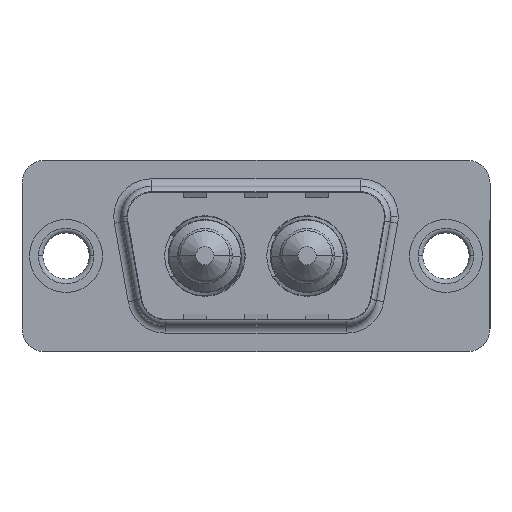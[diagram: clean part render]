
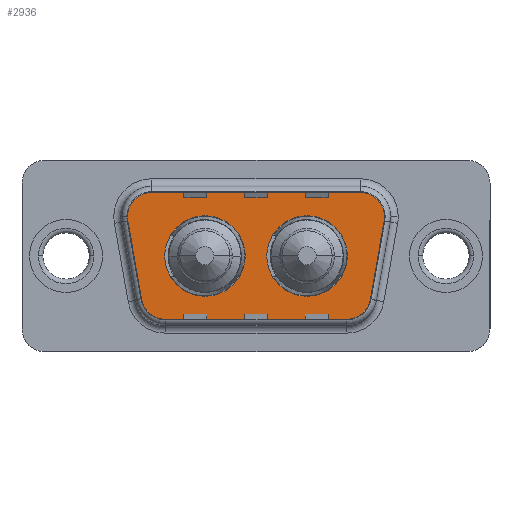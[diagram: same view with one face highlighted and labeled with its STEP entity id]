
A CAD part, top view. The second image highlights one B-rep face of the part: STEP entity #2936.
In plain terms, the highlighted planar face has unit normal (0, 0, 1).
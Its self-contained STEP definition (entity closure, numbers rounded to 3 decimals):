
#11 = CARTESIAN_POINT ( 'NONE',  ( 6.49, 0., 0. ) ) ;
#120 = CIRCLE ( 'NONE', #6072, 2. ) ;
#164 = VERTEX_POINT ( 'NONE', #4654 ) ;
#494 = DIRECTION ( 'NONE',  ( 0., 0., 1. ) ) ;
#540 = CARTESIAN_POINT ( 'NONE',  ( 21.564, 2.9, 0. ) ) ;
#599 = ORIENTED_EDGE ( 'NONE', *, *, #8044, .T. ) ;
#645 = DIRECTION ( 'NONE',  ( 0.174, -0.985, 0. ) ) ;
#717 = DIRECTION ( 'NONE',  ( 1., 0., 0. ) ) ;
#745 = CARTESIAN_POINT ( 'NONE',  ( 18.541, -2.9, 0. ) ) ;
#781 = DIRECTION ( 'NONE',  ( 0., 0., 1. ) ) ;
#797 = DIRECTION ( 'NONE',  ( 1., 0., 0. ) ) ;
#807 = CARTESIAN_POINT ( 'NONE',  ( 5.436, 2.9, 0. ) ) ;
#845 = ORIENTED_EDGE ( 'NONE', *, *, #3369, .T. ) ;
#969 = AXIS2_PLACEMENT_3D ( 'NONE', #7450, #4734, #2533 ) ;
#1001 = VERTEX_POINT ( 'NONE', #7862 ) ;
#1220 = DIRECTION ( 'NONE',  ( 0., 0., 1. ) ) ;
#1245 = ORIENTED_EDGE ( 'NONE', *, *, #6225, .T. ) ;
#1254 = EDGE_LOOP ( 'NONE', ( #5121, #5214 ) ) ;
#1311 = AXIS2_PLACEMENT_3D ( 'NONE', #7008, #5118, #5617 ) ;
#1344 = CARTESIAN_POINT ( 'NONE',  ( 18.541, -2.9, 0. ) ) ;
#1371 = CIRCLE ( 'NONE', #969, 2. ) ;
#1379 = EDGE_CURVE ( 'NONE', #4325, #3999, #5700, .T. ) ;
#1538 = ORIENTED_EDGE ( 'NONE', *, *, #3218, .T. ) ;
#1629 = ORIENTED_EDGE ( 'NONE', *, *, #5001, .T. ) ;
#1735 = AXIS2_PLACEMENT_3D ( 'NONE', #4109, #494, #4221 ) ;
#1847 = DIRECTION ( 'NONE',  ( 0., 0., 1. ) ) ;
#1849 = EDGE_CURVE ( 'NONE', #4382, #5079, #3153, .T. ) ;
#1953 = CIRCLE ( 'NONE', #1735, 2.65 ) ;
#1997 = EDGE_CURVE ( 'NONE', #5298, #2030, #5799, .T. ) ;
#2030 = VERTEX_POINT ( 'NONE', #8335 ) ;
#2045 = CARTESIAN_POINT ( 'NONE',  ( 5.436, 4.9, 0. ) ) ;
#2188 = VECTOR ( 'NONE', #645, 1000. ) ;
#2215 = ORIENTED_EDGE ( 'NONE', *, *, #3448, .T. ) ;
#2357 = CARTESIAN_POINT ( 'NONE',  ( 20.511, -3.247, 0. ) ) ;
#2444 = ORIENTED_EDGE ( 'NONE', *, *, #1379, .T. ) ;
#2533 = DIRECTION ( 'NONE',  ( -1., 0., 0. ) ) ;
#2544 = CIRCLE ( 'NONE', #2766, 2. ) ;
#2592 = DIRECTION ( 'NONE',  ( 0., 0., 1. ) ) ;
#2766 = AXIS2_PLACEMENT_3D ( 'NONE', #6771, #6028, #5940 ) ;
#2767 = DIRECTION ( 'NONE',  ( 1., 0., 0. ) ) ;
#2878 = AXIS2_PLACEMENT_3D ( 'NONE', #3332, #6653, #797 ) ;
#2936 = ADVANCED_FACE ( 'NONE', ( #9308, #7279, #7979 ), #3041, .T. ) ;
#3041 = PLANE ( 'NONE',  #4184 ) ;
#3153 = CIRCLE ( 'NONE', #5623, 2.65 ) ;
#3218 = EDGE_CURVE ( 'NONE', #4404, #4325, #9276, .T. ) ;
#3295 = CARTESIAN_POINT ( 'NONE',  ( 21.534, 2.553, 0. ) ) ;
#3331 = LINE ( 'NONE', #5432, #9616 ) ;
#3332 = CARTESIAN_POINT ( 'NONE',  ( 15.86, 0., 0. ) ) ;
#3369 = EDGE_CURVE ( 'NONE', #7010, #4547, #2544, .T. ) ;
#3393 = CARTESIAN_POINT ( 'NONE',  ( 3.466, 2.553, 0. ) ) ;
#3448 = EDGE_CURVE ( 'NONE', #1001, #3530, #4099, .T. ) ;
#3530 = VERTEX_POINT ( 'NONE', #2045 ) ;
#3618 = DIRECTION ( 'NONE',  ( -1., 0., 0. ) ) ;
#3974 = EDGE_CURVE ( 'NONE', #4547, #164, #3331, .T. ) ;
#3999 = VERTEX_POINT ( 'NONE', #540 ) ;
#4070 = CIRCLE ( 'NONE', #5040, 2. ) ;
#4099 = LINE ( 'NONE', #7490, #5854 ) ;
#4109 = CARTESIAN_POINT ( 'NONE',  ( 15.86, 0., 0. ) ) ;
#4184 = AXIS2_PLACEMENT_3D ( 'NONE', #1344, #1220, #7104 ) ;
#4213 = ORIENTED_EDGE ( 'NONE', *, *, #1997, .F. ) ;
#4221 = DIRECTION ( 'NONE',  ( 1., 0., 0. ) ) ;
#4325 = VERTEX_POINT ( 'NONE', #3295 ) ;
#4382 = VERTEX_POINT ( 'NONE', #11 ) ;
#4395 = LINE ( 'NONE', #9376, #2188 ) ;
#4404 = VERTEX_POINT ( 'NONE', #2357 ) ;
#4547 = VERTEX_POINT ( 'NONE', #4750 ) ;
#4654 = CARTESIAN_POINT ( 'NONE',  ( 18.541, -4.9, 0. ) ) ;
#4734 = DIRECTION ( 'NONE',  ( 0., 0., 1. ) ) ;
#4750 = CARTESIAN_POINT ( 'NONE',  ( 6.459, -4.9, 0. ) ) ;
#5001 = EDGE_CURVE ( 'NONE', #164, #4404, #4070, .T. ) ;
#5009 = AXIS2_PLACEMENT_3D ( 'NONE', #8910, #8559, #3618 ) ;
#5040 = AXIS2_PLACEMENT_3D ( 'NONE', #745, #1847, #7266 ) ;
#5079 = VERTEX_POINT ( 'NONE', #8370 ) ;
#5118 = DIRECTION ( 'NONE',  ( 0., 0., 1. ) ) ;
#5121 = ORIENTED_EDGE ( 'NONE', *, *, #7779, .F. ) ;
#5214 = ORIENTED_EDGE ( 'NONE', *, *, #1849, .F. ) ;
#5298 = VERTEX_POINT ( 'NONE', #7959 ) ;
#5432 = CARTESIAN_POINT ( 'NONE',  ( 6.459, -4.9, 0. ) ) ;
#5617 = DIRECTION ( 'NONE',  ( 1., 0., 0. ) ) ;
#5623 = AXIS2_PLACEMENT_3D ( 'NONE', #8500, #2592, #2767 ) ;
#5652 = EDGE_LOOP ( 'NONE', ( #1629, #1538, #2444, #599, #2215, #1245, #8084, #845, #7962 ) ) ;
#5700 = CIRCLE ( 'NONE', #5009, 2. ) ;
#5759 = DIRECTION ( 'NONE',  ( 0.174, 0.985, 0. ) ) ;
#5799 = CIRCLE ( 'NONE', #2878, 2.65 ) ;
#5854 = VECTOR ( 'NONE', #9096, 1000. ) ;
#5929 = DIRECTION ( 'NONE',  ( 1., 0., 0. ) ) ;
#5940 = DIRECTION ( 'NONE',  ( -1., 0., 0. ) ) ;
#6028 = DIRECTION ( 'NONE',  ( 0., 0., 1. ) ) ;
#6029 = VERTEX_POINT ( 'NONE', #3393 ) ;
#6072 = AXIS2_PLACEMENT_3D ( 'NONE', #807, #781, #717 ) ;
#6225 = EDGE_CURVE ( 'NONE', #3530, #6029, #120, .T. ) ;
#6280 = CARTESIAN_POINT ( 'NONE',  ( 4.489, -3.247, 0. ) ) ;
#6653 = DIRECTION ( 'NONE',  ( 0., 0., 1. ) ) ;
#6771 = CARTESIAN_POINT ( 'NONE',  ( 6.459, -2.9, 0. ) ) ;
#7008 = CARTESIAN_POINT ( 'NONE',  ( 9.14, 0., 0. ) ) ;
#7010 = VERTEX_POINT ( 'NONE', #6280 ) ;
#7021 = EDGE_LOOP ( 'NONE', ( #4213, #9219 ) ) ;
#7104 = DIRECTION ( 'NONE',  ( 1., 0., 0. ) ) ;
#7246 = VECTOR ( 'NONE', #5759, 1000. ) ;
#7266 = DIRECTION ( 'NONE',  ( 1., 0., 0. ) ) ;
#7279 = FACE_BOUND ( 'NONE', #1254, .T. ) ;
#7450 = CARTESIAN_POINT ( 'NONE',  ( 19.564, 2.9, 0. ) ) ;
#7490 = CARTESIAN_POINT ( 'NONE',  ( 5.436, 4.9, 0. ) ) ;
#7638 = CIRCLE ( 'NONE', #1311, 2.65 ) ;
#7779 = EDGE_CURVE ( 'NONE', #5079, #4382, #7638, .T. ) ;
#7862 = CARTESIAN_POINT ( 'NONE',  ( 19.564, 4.9, 0. ) ) ;
#7959 = CARTESIAN_POINT ( 'NONE',  ( 18.51, 0., 0. ) ) ;
#7962 = ORIENTED_EDGE ( 'NONE', *, *, #3974, .T. ) ;
#7979 = FACE_OUTER_BOUND ( 'NONE', #5652, .T. ) ;
#8044 = EDGE_CURVE ( 'NONE', #3999, #1001, #1371, .T. ) ;
#8084 = ORIENTED_EDGE ( 'NONE', *, *, #8164, .T. ) ;
#8164 = EDGE_CURVE ( 'NONE', #6029, #7010, #4395, .T. ) ;
#8261 = EDGE_CURVE ( 'NONE', #2030, #5298, #1953, .T. ) ;
#8335 = CARTESIAN_POINT ( 'NONE',  ( 13.21, 0., 0. ) ) ;
#8370 = CARTESIAN_POINT ( 'NONE',  ( 11.79, 0., 0. ) ) ;
#8500 = CARTESIAN_POINT ( 'NONE',  ( 9.14, 0., 0. ) ) ;
#8559 = DIRECTION ( 'NONE',  ( 0., 0., 1. ) ) ;
#8832 = CARTESIAN_POINT ( 'NONE',  ( 21.534, 2.553, 0. ) ) ;
#8910 = CARTESIAN_POINT ( 'NONE',  ( 19.564, 2.9, 0. ) ) ;
#9096 = DIRECTION ( 'NONE',  ( -1., 0., 0. ) ) ;
#9219 = ORIENTED_EDGE ( 'NONE', *, *, #8261, .F. ) ;
#9276 = LINE ( 'NONE', #8832, #7246 ) ;
#9308 = FACE_BOUND ( 'NONE', #7021, .T. ) ;
#9376 = CARTESIAN_POINT ( 'NONE',  ( 3.466, 2.553, 0. ) ) ;
#9616 = VECTOR ( 'NONE', #5929, 1000. ) ;
